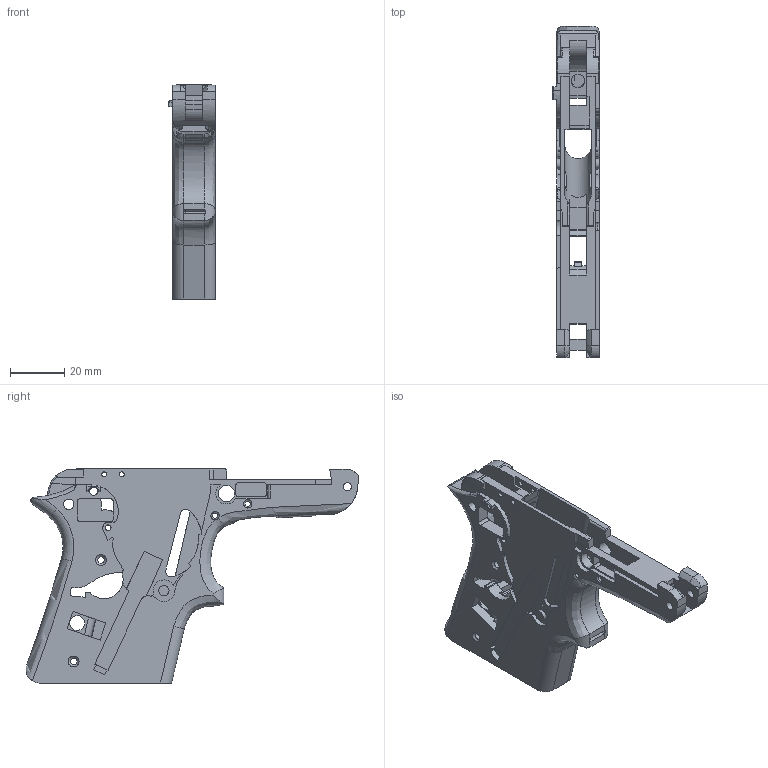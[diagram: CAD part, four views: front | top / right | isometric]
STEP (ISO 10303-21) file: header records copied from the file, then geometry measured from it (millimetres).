
FILE_DESCRIPTION(/* description */ (''),/* implementation_level */ '2;1');
FILE_NAME(/* name */ '21a v1.0.step',/* time_stamp */ '2021-11-23T22:27:24-05:00',/* author */ (''),/* organization */ (''),/* preprocessor_version */ 'ST-DEVELOPER v18.1',/* originating_system */ 'Autodesk Translation Framework v10.10.0.1391',/* authorisation */ '');
FILE_SCHEMA (('AUTOMOTIVE_DESIGN { 1 0 10303 214 3 1 1 }'));
Products named in the file (2): barrel; frame
Assembly tree (1 placements, depth 2):
  barrel
    frame
Bounding box: 17.2 x 122.46 x 78.94 mm (x, y, z)
Volume: 40984 mm3; surface area: 25959.3 mm2
Topology: 1 solids, 1 shells, 1133 faces, 3292 edges, 2186 vertices
Faces by surface type: bspline 716, plane 255, cylinder 139, torus 16, cone 5, sphere 2
Full cylindrical faces by diameter (mm): 1.8 x4, 2.05 x2, 2.1 x2, 2.14 x2, 2.5 x3, 2.98 x2, 3 x2, 3.8 x4, 5 x1, 5.5 x1, 6.1 x2, 8.7 x1
Entity records: 43439 total; most frequent: CARTESIAN_POINT 20377, ORIENTED_EDGE 6580, EDGE_CURVE 3290, DIRECTION 2800, VERTEX_POINT 2186, LINE 1328, VECTOR 1328, EDGE_LOOP 1228
